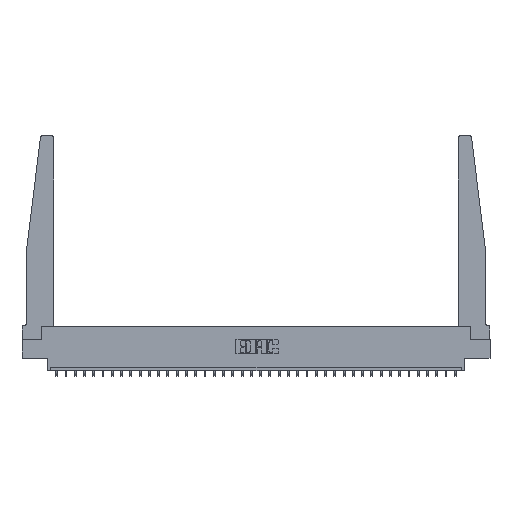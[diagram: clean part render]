
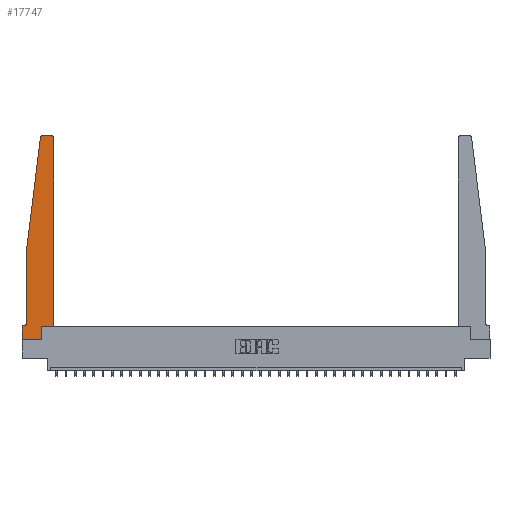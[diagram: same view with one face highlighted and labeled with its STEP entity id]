
A CAD part, top view. The second image highlights one B-rep face of the part: STEP entity #17747.
In plain terms, the highlighted planar face has unit normal (0, 0, 1).
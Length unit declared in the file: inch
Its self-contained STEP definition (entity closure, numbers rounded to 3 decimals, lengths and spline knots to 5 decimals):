
#168 = EDGE_CURVE ( 'NONE', #19000, #27974, #2212, .T. ) ;
#492 = DIRECTION ( 'NONE',  ( 0., 0., 1. ) ) ;
#684 = CARTESIAN_POINT ( 'NONE',  ( 0., 0., 0.37 ) ) ;
#1065 = DIRECTION ( 'NONE',  ( -1., 0., 0. ) ) ;
#2212 = CIRCLE ( 'NONE', #20584, 0.05 ) ;
#2677 = EDGE_CURVE ( 'NONE', #2736, #29728, #22786, .T. ) ;
#2736 = VERTEX_POINT ( 'NONE', #16326 ) ;
#2889 = DIRECTION ( 'NONE',  ( 0., 1., 0. ) ) ;
#2988 = DIRECTION ( 'NONE',  ( 1., 0., 0. ) ) ;
#3076 = VECTOR ( 'NONE', #29893, 39.37008 ) ;
#3857 = AXIS2_PLACEMENT_3D ( 'NONE', #25046, #20276, #10043 ) ;
#3879 = VECTOR ( 'NONE', #22693, 39.37008 ) ;
#4951 = CARTESIAN_POINT ( 'NONE',  ( 0.2605, 0., 0.37 ) ) ;
#5741 = LINE ( 'NONE', #20856, #3879 ) ;
#5770 = LINE ( 'NONE', #684, #15196 ) ;
#6973 = ORIENTED_EDGE ( 'NONE', *, *, #21986, .T. ) ;
#7057 = EDGE_CURVE ( 'NONE', #24730, #19294, #5770, .T. ) ;
#7191 = EDGE_CURVE ( 'NONE', #19294, #31344, #22889, .T. ) ;
#7389 = DIRECTION ( 'NONE',  ( 1., 0., 0. ) ) ;
#7464 = CARTESIAN_POINT ( 'NONE',  ( 0.065, 1.25, 0.37 ) ) ;
#7621 = DIRECTION ( 'NONE',  ( 0., 0., 1. ) ) ;
#7877 = CARTESIAN_POINT ( 'NONE',  ( 0.395, 2.72, 0.37 ) ) ;
#8544 = EDGE_CURVE ( 'NONE', #31344, #2736, #12652, .T. ) ;
#8610 = EDGE_CURVE ( 'NONE', #11057, #24730, #9511, .T. ) ;
#8914 = LINE ( 'NONE', #16030, #10610 ) ;
#9402 = ORIENTED_EDGE ( 'NONE', *, *, #8610, .T. ) ;
#9511 = LINE ( 'NONE', #9675, #3076 ) ;
#9675 = CARTESIAN_POINT ( 'NONE',  ( 0., 0., 0.37 ) ) ;
#10043 = DIRECTION ( 'NONE',  ( 1., 0., 0. ) ) ;
#10400 = VERTEX_POINT ( 'NONE', #30392 ) ;
#10610 = VECTOR ( 'NONE', #1065, 39.37008 ) ;
#10847 = ORIENTED_EDGE ( 'NONE', *, *, #168, .T. ) ;
#11057 = VERTEX_POINT ( 'NONE', #14224 ) ;
#12065 = LINE ( 'NONE', #7464, #29825 ) ;
#12179 = EDGE_CURVE ( 'NONE', #27974, #11057, #23468, .T. ) ;
#12249 = CIRCLE ( 'NONE', #16433, 0.03 ) ;
#12652 = LINE ( 'NONE', #15100, #22506 ) ;
#13168 = DIRECTION ( 'NONE',  ( 0., 1., 0. ) ) ;
#13760 = ORIENTED_EDGE ( 'NONE', *, *, #7057, .T. ) ;
#13767 = CIRCLE ( 'NONE', #32142, 0.03 ) ;
#13852 = ORIENTED_EDGE ( 'NONE', *, *, #2677, .T. ) ;
#14063 = CARTESIAN_POINT ( 'NONE',  ( 0.065, 0.1875, 0.37 ) ) ;
#14224 = CARTESIAN_POINT ( 'NONE',  ( 0., 0.1875, 0.37 ) ) ;
#14976 = EDGE_CURVE ( 'NONE', #24206, #24367, #8914, .T. ) ;
#14991 = PLANE ( 'NONE',  #3857 ) ;
#15100 = CARTESIAN_POINT ( 'NONE',  ( 0.425, 0.18, 0.37 ) ) ;
#15196 = VECTOR ( 'NONE', #2988, 39.37008 ) ;
#15349 = EDGE_CURVE ( 'NONE', #24367, #30786, #12249, .T. ) ;
#16030 = CARTESIAN_POINT ( 'NONE',  ( 0.25, 2.75, 0.37 ) ) ;
#16326 = CARTESIAN_POINT ( 'NONE',  ( 0.425, 0.18, 0.37 ) ) ;
#16433 = AXIS2_PLACEMENT_3D ( 'NONE', #27528, #7621, #20447 ) ;
#16446 = CARTESIAN_POINT ( 'NONE',  ( 0.425, 2.72, 0.37 ) ) ;
#16779 = DIRECTION ( 'NONE',  ( 0., 0., -1. ) ) ;
#17054 = ORIENTED_EDGE ( 'NONE', *, *, #17143, .T. ) ;
#17143 = EDGE_CURVE ( 'NONE', #29728, #24206, #13767, .T. ) ;
#17516 = DIRECTION ( 'NONE',  ( -0.122, -0.992, 0. ) ) ;
#17649 = CARTESIAN_POINT ( 'NONE',  ( 0., 0., 0.37 ) ) ;
#17747 = ADVANCED_FACE ( 'NONE', ( #27670 ), #14991, .T. ) ;
#18261 = EDGE_CURVE ( 'NONE', #10400, #19000, #5741, .T. ) ;
#18367 = VECTOR ( 'NONE', #13168, 39.37008 ) ;
#19000 = VERTEX_POINT ( 'NONE', #30423 ) ;
#19032 = DIRECTION ( 'NONE',  ( -1., 0., 0. ) ) ;
#19294 = VERTEX_POINT ( 'NONE', #4951 ) ;
#19986 = CARTESIAN_POINT ( 'NONE',  ( 0.395, 2.75, 0.37 ) ) ;
#20276 = DIRECTION ( 'NONE',  ( 0., 0., 1. ) ) ;
#20447 = DIRECTION ( 'NONE',  ( 1., 0., 0. ) ) ;
#20573 = CARTESIAN_POINT ( 'NONE',  ( 0.2605, 0.18, 0.37 ) ) ;
#20584 = AXIS2_PLACEMENT_3D ( 'NONE', #29589, #16779, #31709 ) ;
#20856 = CARTESIAN_POINT ( 'NONE',  ( 0.065, 1.25, 0.37 ) ) ;
#21986 = EDGE_CURVE ( 'NONE', #30786, #10400, #12065, .T. ) ;
#22323 = ORIENTED_EDGE ( 'NONE', *, *, #7191, .T. ) ;
#22506 = VECTOR ( 'NONE', #7389, 39.37008 ) ;
#22693 = DIRECTION ( 'NONE',  ( 0., -1., 0. ) ) ;
#22786 = LINE ( 'NONE', #22949, #30368 ) ;
#22889 = LINE ( 'NONE', #20573, #18367 ) ;
#22949 = CARTESIAN_POINT ( 'NONE',  ( 0.425, 0.18, 0.37 ) ) ;
#23132 = ORIENTED_EDGE ( 'NONE', *, *, #12179, .T. ) ;
#23468 = LINE ( 'NONE', #14063, #26245 ) ;
#23824 = ORIENTED_EDGE ( 'NONE', *, *, #8544, .T. ) ;
#24037 = ORIENTED_EDGE ( 'NONE', *, *, #14976, .T. ) ;
#24206 = VERTEX_POINT ( 'NONE', #19986 ) ;
#24367 = VERTEX_POINT ( 'NONE', #30620 ) ;
#24730 = VERTEX_POINT ( 'NONE', #17649 ) ;
#25046 = CARTESIAN_POINT ( 'NONE',  ( 0., 0.1875, 0.37 ) ) ;
#25704 = CARTESIAN_POINT ( 'NONE',  ( 0.015, 0.1875, 0.37 ) ) ;
#26162 = CARTESIAN_POINT ( 'NONE',  ( 0.24675, 2.72367, 0.37 ) ) ;
#26245 = VECTOR ( 'NONE', #19032, 39.37008 ) ;
#27095 = EDGE_LOOP ( 'NONE', ( #24037, #31437, #6973, #31849, #10847, #23132, #9402, #13760, #22323, #23824, #13852, #17054 ) ) ;
#27528 = CARTESIAN_POINT ( 'NONE',  ( 0.27653, 2.72, 0.37 ) ) ;
#27670 = FACE_OUTER_BOUND ( 'NONE', #27095, .T. ) ;
#27974 = VERTEX_POINT ( 'NONE', #25704 ) ;
#29589 = CARTESIAN_POINT ( 'NONE',  ( 0.015, 0.2375, 0.37 ) ) ;
#29728 = VERTEX_POINT ( 'NONE', #16446 ) ;
#29825 = VECTOR ( 'NONE', #17516, 39.37008 ) ;
#29893 = DIRECTION ( 'NONE',  ( 0., -1., 0. ) ) ;
#30052 = DIRECTION ( 'NONE',  ( 1., 0., 0. ) ) ;
#30368 = VECTOR ( 'NONE', #2889, 39.37008 ) ;
#30392 = CARTESIAN_POINT ( 'NONE',  ( 0.065, 1.25, 0.37 ) ) ;
#30423 = CARTESIAN_POINT ( 'NONE',  ( 0.065, 0.2375, 0.37 ) ) ;
#30620 = CARTESIAN_POINT ( 'NONE',  ( 0.27653, 2.75, 0.37 ) ) ;
#30786 = VERTEX_POINT ( 'NONE', #26162 ) ;
#31344 = VERTEX_POINT ( 'NONE', #31505 ) ;
#31437 = ORIENTED_EDGE ( 'NONE', *, *, #15349, .T. ) ;
#31505 = CARTESIAN_POINT ( 'NONE',  ( 0.2605, 0.18, 0.37 ) ) ;
#31709 = DIRECTION ( 'NONE',  ( -1., 0., 0. ) ) ;
#31849 = ORIENTED_EDGE ( 'NONE', *, *, #18261, .T. ) ;
#32142 = AXIS2_PLACEMENT_3D ( 'NONE', #7877, #492, #30052 ) ;
